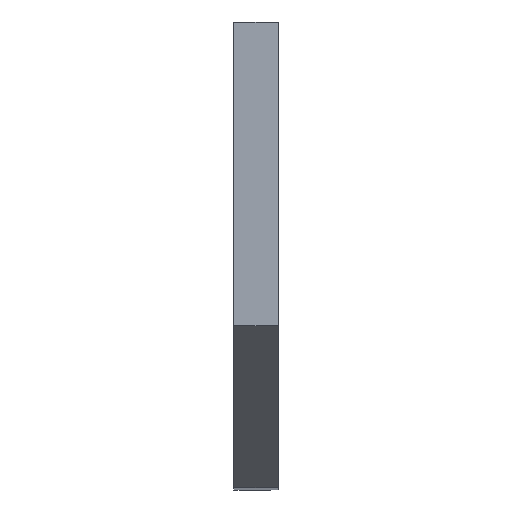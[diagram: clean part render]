
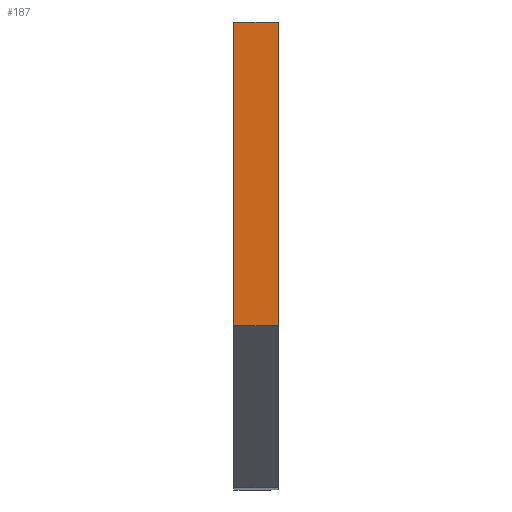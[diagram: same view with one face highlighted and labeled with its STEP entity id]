
A CAD part, top view. The second image highlights one B-rep face of the part: STEP entity #187.
In plain terms, the highlighted planar face has unit normal (0, 0, 1).
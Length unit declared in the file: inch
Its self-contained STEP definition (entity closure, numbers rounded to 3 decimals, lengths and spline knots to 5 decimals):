
#44 = ORIENTED_EDGE ( 'NONE', *, *, #79, .F. ) ;
#51 = PLANE ( 'NONE',  #542 ) ;
#53 = VERTEX_POINT ( 'NONE', #255 ) ;
#79 = EDGE_CURVE ( 'NONE', #355, #694, #1040, .T. ) ;
#81 = EDGE_CURVE ( 'NONE', #53, #253, #1276, .T. ) ;
#187 = ADVANCED_FACE ( 'NONE', ( #946 ), #51, .T. ) ;
#248 = VECTOR ( 'NONE', #499, 39.37008 ) ;
#253 = VERTEX_POINT ( 'NONE', #959 ) ;
#255 = CARTESIAN_POINT ( 'NONE',  ( -0.125, 1.316, 0. ) ) ;
#355 = VERTEX_POINT ( 'NONE', #609 ) ;
#423 = EDGE_LOOP ( 'NONE', ( #44, #602, #972, #1088 ) ) ;
#489 = LINE ( 'NONE', #1160, #1200 ) ;
#499 = DIRECTION ( 'NONE',  ( 0., -1., 0. ) ) ;
#502 = CARTESIAN_POINT ( 'NONE',  ( -0.125, 0., 0. ) ) ;
#536 = VECTOR ( 'NONE', #1277, 39.37008 ) ;
#542 = AXIS2_PLACEMENT_3D ( 'NONE', #1255, #838, #650 ) ;
#554 = DIRECTION ( 'NONE',  ( 1., 0., 0. ) ) ;
#602 = ORIENTED_EDGE ( 'NONE', *, *, #1196, .F. ) ;
#609 = CARTESIAN_POINT ( 'NONE',  ( 0., 1.316, 0. ) ) ;
#650 = DIRECTION ( 'NONE',  ( 0., -1., 0. ) ) ;
#694 = VERTEX_POINT ( 'NONE', #1201 ) ;
#723 = CARTESIAN_POINT ( 'NONE',  ( 0., 0., 0. ) ) ;
#767 = CARTESIAN_POINT ( 'NONE',  ( -0.125, 0.457, 0. ) ) ;
#802 = LINE ( 'NONE', #767, #536 ) ;
#828 = VECTOR ( 'NONE', #911, 39.37008 ) ;
#838 = DIRECTION ( 'NONE',  ( 0., 0., 1. ) ) ;
#911 = DIRECTION ( 'NONE',  ( 0., -1., 0. ) ) ;
#946 = FACE_OUTER_BOUND ( 'NONE', #423, .T. ) ;
#959 = CARTESIAN_POINT ( 'NONE',  ( -0.125, 0.457, 0. ) ) ;
#972 = ORIENTED_EDGE ( 'NONE', *, *, #81, .T. ) ;
#1040 = LINE ( 'NONE', #723, #828 ) ;
#1088 = ORIENTED_EDGE ( 'NONE', *, *, #1282, .T. ) ;
#1160 = CARTESIAN_POINT ( 'NONE',  ( -0.125, 1.316, 0. ) ) ;
#1196 = EDGE_CURVE ( 'NONE', #53, #355, #489, .T. ) ;
#1200 = VECTOR ( 'NONE', #554, 39.37008 ) ;
#1201 = CARTESIAN_POINT ( 'NONE',  ( 0., 0.457, 0. ) ) ;
#1255 = CARTESIAN_POINT ( 'NONE',  ( -0.125, 0., 0. ) ) ;
#1276 = LINE ( 'NONE', #502, #248 ) ;
#1277 = DIRECTION ( 'NONE',  ( 1., 0., 0. ) ) ;
#1282 = EDGE_CURVE ( 'NONE', #253, #694, #802, .T. ) ;
